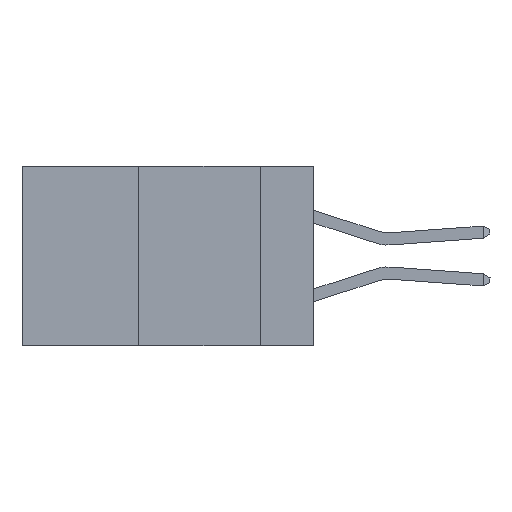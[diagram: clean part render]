
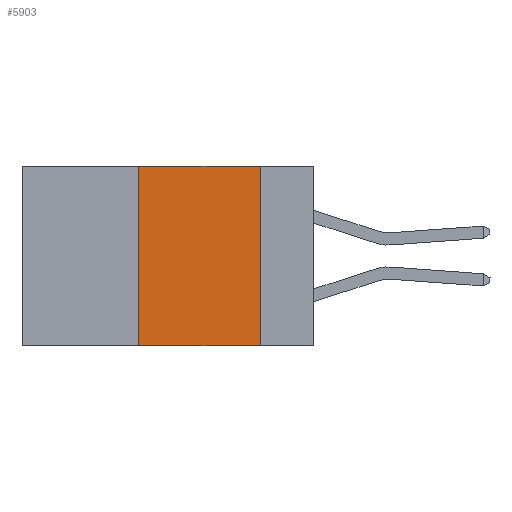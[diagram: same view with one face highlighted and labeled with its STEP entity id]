
A CAD part, left-side view. The second image highlights one B-rep face of the part: STEP entity #5903.
In plain terms, the highlighted planar face has unit normal (-1, 0, 0).
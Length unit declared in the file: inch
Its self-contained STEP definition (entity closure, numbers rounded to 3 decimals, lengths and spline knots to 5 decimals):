
#360 = LINE ( 'NONE', #7287, #12419 ) ;
#946 = EDGE_CURVE ( 'NONE', #12281, #7661, #5333, .T. ) ;
#1120 = DIRECTION ( 'NONE',  ( 0., -1., 0. ) ) ;
#1520 = DIRECTION ( 'NONE',  ( 0., -1., 0. ) ) ;
#2068 = VECTOR ( 'NONE', #1520, 39.37008 ) ;
#2525 = CARTESIAN_POINT ( 'NONE',  ( 0., 0.11, -0.37 ) ) ;
#3111 = DIRECTION ( 'NONE',  ( 0., 0., -1. ) ) ;
#3198 = DIRECTION ( 'NONE',  ( 1., 0., 0. ) ) ;
#3370 = AXIS2_PLACEMENT_3D ( 'NONE', #11829, #3198, #3111 ) ;
#3434 = CARTESIAN_POINT ( 'NONE',  ( 0., 0.6, 0. ) ) ;
#3732 = EDGE_LOOP ( 'NONE', ( #6539, #6809, #13173, #9263 ) ) ;
#4536 = EDGE_CURVE ( 'NONE', #5011, #9627, #12105, .T. ) ;
#4640 = FACE_OUTER_BOUND ( 'NONE', #3732, .T. ) ;
#4871 = CARTESIAN_POINT ( 'NONE',  ( 0., 0.36, -0.37 ) ) ;
#5011 = VERTEX_POINT ( 'NONE', #13856 ) ;
#5333 = LINE ( 'NONE', #6929, #2068 ) ;
#5903 = ADVANCED_FACE ( 'NONE', ( #4640 ), #13991, .F. ) ;
#6539 = ORIENTED_EDGE ( 'NONE', *, *, #8699, .F. ) ;
#6799 = CARTESIAN_POINT ( 'NONE',  ( 0., 0.11, 0. ) ) ;
#6809 = ORIENTED_EDGE ( 'NONE', *, *, #4536, .F. ) ;
#6929 = CARTESIAN_POINT ( 'NONE',  ( 0., 0.6, -0.37 ) ) ;
#7287 = CARTESIAN_POINT ( 'NONE',  ( 0., 0.36, 0. ) ) ;
#7471 = DIRECTION ( 'NONE',  ( 0., 0., 1. ) ) ;
#7661 = VERTEX_POINT ( 'NONE', #2525 ) ;
#8164 = VECTOR ( 'NONE', #10813, 39.37008 ) ;
#8699 = EDGE_CURVE ( 'NONE', #9627, #7661, #10209, .T. ) ;
#9263 = ORIENTED_EDGE ( 'NONE', *, *, #946, .T. ) ;
#9627 = VERTEX_POINT ( 'NONE', #6799 ) ;
#10166 = VECTOR ( 'NONE', #1120, 39.37008 ) ;
#10209 = LINE ( 'NONE', #10719, #8164 ) ;
#10719 = CARTESIAN_POINT ( 'NONE',  ( 0., 0.11, 0. ) ) ;
#10813 = DIRECTION ( 'NONE',  ( 0., 0., -1. ) ) ;
#11375 = EDGE_CURVE ( 'NONE', #12281, #5011, #360, .T. ) ;
#11829 = CARTESIAN_POINT ( 'NONE',  ( 0., 0.6, 0. ) ) ;
#12105 = LINE ( 'NONE', #3434, #10166 ) ;
#12281 = VERTEX_POINT ( 'NONE', #4871 ) ;
#12419 = VECTOR ( 'NONE', #7471, 39.37008 ) ;
#13173 = ORIENTED_EDGE ( 'NONE', *, *, #11375, .F. ) ;
#13856 = CARTESIAN_POINT ( 'NONE',  ( 0., 0.36, 0. ) ) ;
#13991 = PLANE ( 'NONE',  #3370 ) ;
